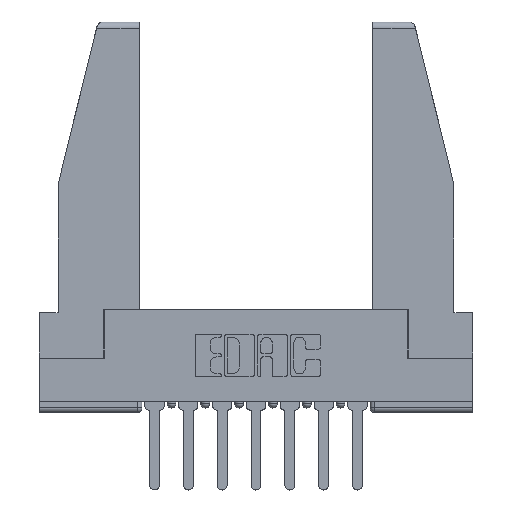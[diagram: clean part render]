
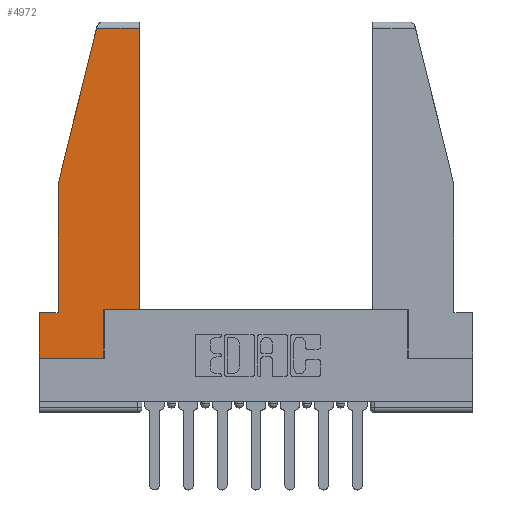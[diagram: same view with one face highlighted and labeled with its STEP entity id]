
A CAD part, top view. The second image highlights one B-rep face of the part: STEP entity #4972.
In plain terms, the highlighted planar face has unit normal (0, 0, 1).
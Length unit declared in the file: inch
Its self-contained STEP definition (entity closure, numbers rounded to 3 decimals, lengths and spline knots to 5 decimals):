
#351 = CARTESIAN_POINT ( 'NONE',  ( 0.297, 0., 0. ) ) ;
#1378 = DIRECTION ( 'NONE',  ( -1., 0., 0. ) ) ;
#1401 = DIRECTION ( 'NONE',  ( 0., 1., 0. ) ) ;
#1450 = EDGE_CURVE ( 'NONE', #12868, #6228, #12401, .T. ) ;
#1561 = PLANE ( 'NONE',  #11205 ) ;
#1667 = LINE ( 'NONE', #9133, #6382 ) ;
#1729 = VERTEX_POINT ( 'NONE', #6312 ) ;
#2366 = VERTEX_POINT ( 'NONE', #5796 ) ;
#2534 = EDGE_CURVE ( 'NONE', #10560, #5427, #3119, .T. ) ;
#2687 = VERTEX_POINT ( 'NONE', #5606 ) ;
#2906 = LINE ( 'NONE', #7613, #11547 ) ;
#3101 = VERTEX_POINT ( 'NONE', #10292 ) ;
#3119 = LINE ( 'NONE', #8266, #4544 ) ;
#3660 = VERTEX_POINT ( 'NONE', #7104 ) ;
#3767 = CARTESIAN_POINT ( 'NONE',  ( 0., 0., 0. ) ) ;
#3943 = CARTESIAN_POINT ( 'NONE',  ( 0.2636, 1.52, 0. ) ) ;
#4045 = ORIENTED_EDGE ( 'NONE', *, *, #6570, .T. ) ;
#4084 = LINE ( 'NONE', #3767, #5041 ) ;
#4381 = DIRECTION ( 'NONE',  ( -0.239, -0.971, 0. ) ) ;
#4544 = VECTOR ( 'NONE', #4381, 39.37008 ) ;
#4972 = ADVANCED_FACE ( 'NONE', ( #6858 ), #1561, .T. ) ;
#5041 = VECTOR ( 'NONE', #8726, 39.37008 ) ;
#5110 = DIRECTION ( 'NONE',  ( 0., -1., 0. ) ) ;
#5115 = CARTESIAN_POINT ( 'NONE',  ( 0.297, 0., 0. ) ) ;
#5179 = EDGE_CURVE ( 'NONE', #3660, #2366, #10943, .T. ) ;
#5427 = VERTEX_POINT ( 'NONE', #12539 ) ;
#5606 = CARTESIAN_POINT ( 'NONE',  ( 0.086, 0.21, 0. ) ) ;
#5735 = CARTESIAN_POINT ( 'NONE',  ( 0.086, 0.8, 0. ) ) ;
#5796 = CARTESIAN_POINT ( 'NONE',  ( 0., 0., 0. ) ) ;
#6157 = ORIENTED_EDGE ( 'NONE', *, *, #5179, .T. ) ;
#6228 = VERTEX_POINT ( 'NONE', #8741 ) ;
#6312 = CARTESIAN_POINT ( 'NONE',  ( 0.461, 0.223, 0. ) ) ;
#6370 = CARTESIAN_POINT ( 'NONE',  ( 0., 1.52, 0. ) ) ;
#6382 = VECTOR ( 'NONE', #7204, 39.37008 ) ;
#6570 = EDGE_CURVE ( 'NONE', #2687, #3660, #1667, .T. ) ;
#6598 = VECTOR ( 'NONE', #1401, 39.37008 ) ;
#6858 = FACE_OUTER_BOUND ( 'NONE', #11885, .T. ) ;
#6862 = ORIENTED_EDGE ( 'NONE', *, *, #9364, .T. ) ;
#7104 = CARTESIAN_POINT ( 'NONE',  ( 0., 0.21, 0. ) ) ;
#7204 = DIRECTION ( 'NONE',  ( -1., 0., 0. ) ) ;
#7613 = CARTESIAN_POINT ( 'NONE',  ( 0.297, 0.223, 0. ) ) ;
#8118 = EDGE_CURVE ( 'NONE', #3101, #10560, #8341, .T. ) ;
#8159 = VECTOR ( 'NONE', #10135, 39.37008 ) ;
#8266 = CARTESIAN_POINT ( 'NONE',  ( 0.271, 1.55, 0. ) ) ;
#8296 = CARTESIAN_POINT ( 'NONE',  ( 0.461, 0.223, 0. ) ) ;
#8341 = LINE ( 'NONE', #6370, #12128 ) ;
#8359 = ORIENTED_EDGE ( 'NONE', *, *, #8118, .T. ) ;
#8452 = CARTESIAN_POINT ( 'NONE',  ( 0., 0., 0. ) ) ;
#8639 = DIRECTION ( 'NONE',  ( 0., -1., 0. ) ) ;
#8726 = DIRECTION ( 'NONE',  ( 1., 0., 0. ) ) ;
#8741 = CARTESIAN_POINT ( 'NONE',  ( 0.297, 0.223, 0. ) ) ;
#8864 = CARTESIAN_POINT ( 'NONE',  ( 0., 0.21, 0. ) ) ;
#9023 = LINE ( 'NONE', #5735, #9964 ) ;
#9133 = CARTESIAN_POINT ( 'NONE',  ( 0., 0.21, 0. ) ) ;
#9364 = EDGE_CURVE ( 'NONE', #1729, #3101, #11786, .T. ) ;
#9571 = DIRECTION ( 'NONE',  ( 1., 0., 0. ) ) ;
#9586 = EDGE_CURVE ( 'NONE', #2366, #12868, #4084, .T. ) ;
#9964 = VECTOR ( 'NONE', #8639, 39.37008 ) ;
#10107 = ORIENTED_EDGE ( 'NONE', *, *, #11670, .T. ) ;
#10135 = DIRECTION ( 'NONE',  ( 0., 1., 0. ) ) ;
#10292 = CARTESIAN_POINT ( 'NONE',  ( 0.461, 1.52, 0. ) ) ;
#10560 = VERTEX_POINT ( 'NONE', #3943 ) ;
#10943 = LINE ( 'NONE', #8864, #11570 ) ;
#11205 = AXIS2_PLACEMENT_3D ( 'NONE', #8452, #12411, #9571 ) ;
#11329 = ORIENTED_EDGE ( 'NONE', *, *, #1450, .T. ) ;
#11547 = VECTOR ( 'NONE', #11655, 39.37008 ) ;
#11570 = VECTOR ( 'NONE', #5110, 39.37008 ) ;
#11655 = DIRECTION ( 'NONE',  ( 1., 0., 0. ) ) ;
#11670 = EDGE_CURVE ( 'NONE', #6228, #1729, #2906, .T. ) ;
#11736 = EDGE_CURVE ( 'NONE', #5427, #2687, #9023, .T. ) ;
#11786 = LINE ( 'NONE', #8296, #6598 ) ;
#11885 = EDGE_LOOP ( 'NONE', ( #6862, #8359, #12922, #12273, #4045, #6157, #12023, #11329, #10107 ) ) ;
#12023 = ORIENTED_EDGE ( 'NONE', *, *, #9586, .T. ) ;
#12128 = VECTOR ( 'NONE', #1378, 39.37008 ) ;
#12273 = ORIENTED_EDGE ( 'NONE', *, *, #11736, .T. ) ;
#12401 = LINE ( 'NONE', #5115, #8159 ) ;
#12411 = DIRECTION ( 'NONE',  ( 0., 0., 1. ) ) ;
#12539 = CARTESIAN_POINT ( 'NONE',  ( 0.086, 0.8, 0. ) ) ;
#12868 = VERTEX_POINT ( 'NONE', #351 ) ;
#12922 = ORIENTED_EDGE ( 'NONE', *, *, #2534, .T. ) ;
